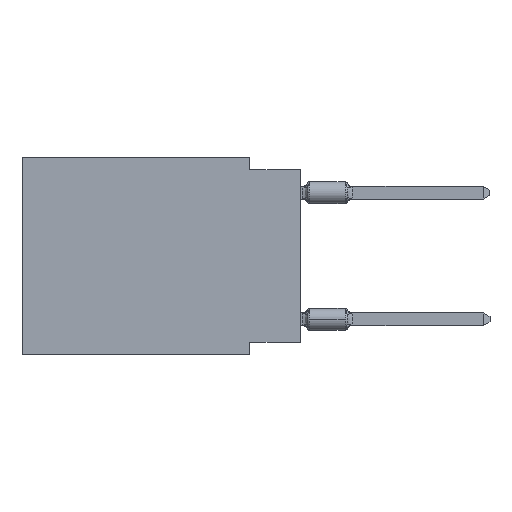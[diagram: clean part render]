
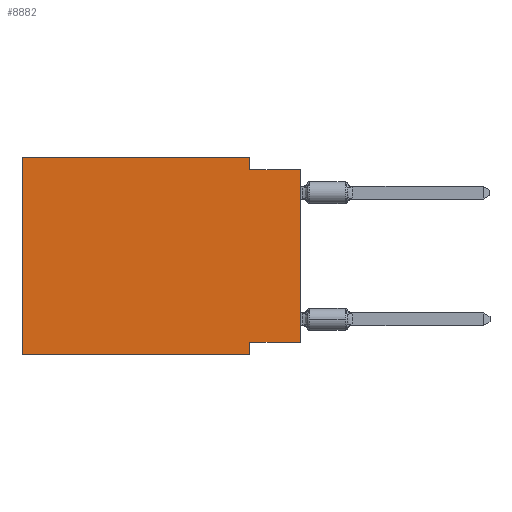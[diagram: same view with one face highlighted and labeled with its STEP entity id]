
A CAD part, left-side view. The second image highlights one B-rep face of the part: STEP entity #8882.
In plain terms, the highlighted planar face has unit normal (-1, 0, 0).
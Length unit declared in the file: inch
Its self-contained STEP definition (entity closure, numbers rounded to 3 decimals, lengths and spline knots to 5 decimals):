
#130 = EDGE_CURVE ( 'NONE', #8634, #6381, #14259, .T. ) ;
#194 = EDGE_CURVE ( 'NONE', #8634, #4099, #12026, .T. ) ;
#901 = EDGE_CURVE ( 'NONE', #6381, #3580, #13754, .T. ) ;
#1161 = VERTEX_POINT ( 'NONE', #1601 ) ;
#1203 = LINE ( 'NONE', #8480, #13628 ) ;
#1282 = EDGE_CURVE ( 'NONE', #3580, #2836, #10297, .T. ) ;
#1601 = CARTESIAN_POINT ( 'NONE',  ( 0., 0.1, -0.365 ) ) ;
#1873 = VECTOR ( 'NONE', #9549, 39.37008 ) ;
#1972 = ORIENTED_EDGE ( 'NONE', *, *, #6650, .F. ) ;
#2029 = VECTOR ( 'NONE', #4628, 39.37008 ) ;
#2389 = AXIS2_PLACEMENT_3D ( 'NONE', #9356, #9590, #9273 ) ;
#2646 = CARTESIAN_POINT ( 'NONE',  ( 0., 0., -0.025 ) ) ;
#2836 = VERTEX_POINT ( 'NONE', #4512 ) ;
#3253 = DIRECTION ( 'NONE',  ( 0., 0., 1. ) ) ;
#3470 = VECTOR ( 'NONE', #3253, 39.37008 ) ;
#3580 = VERTEX_POINT ( 'NONE', #4321 ) ;
#4099 = VERTEX_POINT ( 'NONE', #14002 ) ;
#4321 = CARTESIAN_POINT ( 'NONE',  ( 0., 0.1, 0. ) ) ;
#4357 = CARTESIAN_POINT ( 'NONE',  ( 0., 0.55, 0. ) ) ;
#4377 = CARTESIAN_POINT ( 'NONE',  ( 0., 0., 0. ) ) ;
#4426 = VERTEX_POINT ( 'NONE', #13079 ) ;
#4475 = CARTESIAN_POINT ( 'NONE',  ( 0., 0.1, 0. ) ) ;
#4512 = CARTESIAN_POINT ( 'NONE',  ( 0., 0.1, -0.025 ) ) ;
#4529 = VECTOR ( 'NONE', #9880, 39.37008 ) ;
#4559 = EDGE_CURVE ( 'NONE', #2836, #14212, #1203, .T. ) ;
#4628 = DIRECTION ( 'NONE',  ( 0., -1., 0. ) ) ;
#5025 = CARTESIAN_POINT ( 'NONE',  ( 0., 0.1, -0.39 ) ) ;
#5180 = EDGE_CURVE ( 'NONE', #4426, #14212, #15521, .T. ) ;
#5213 = EDGE_LOOP ( 'NONE', ( #6523, #6225, #11697, #9829, #9132, #13107, #1972, #9410 ) ) ;
#6225 = ORIENTED_EDGE ( 'NONE', *, *, #4559, .F. ) ;
#6381 = VERTEX_POINT ( 'NONE', #9246 ) ;
#6523 = ORIENTED_EDGE ( 'NONE', *, *, #5180, .T. ) ;
#6650 = EDGE_CURVE ( 'NONE', #1161, #4099, #11060, .T. ) ;
#7401 = VECTOR ( 'NONE', #12105, 39.37008 ) ;
#8480 = CARTESIAN_POINT ( 'NONE',  ( 0., 0., -0.025 ) ) ;
#8535 = CARTESIAN_POINT ( 'NONE',  ( 0., 0.55, 0. ) ) ;
#8634 = VERTEX_POINT ( 'NONE', #14031 ) ;
#8882 = ADVANCED_FACE ( 'NONE', ( #15630 ), #15552, .F. ) ;
#9132 = ORIENTED_EDGE ( 'NONE', *, *, #130, .F. ) ;
#9220 = DIRECTION ( 'NONE',  ( 0., -1., 0. ) ) ;
#9246 = CARTESIAN_POINT ( 'NONE',  ( 0., 0.55, 0. ) ) ;
#9273 = DIRECTION ( 'NONE',  ( 0., 0., -1. ) ) ;
#9356 = CARTESIAN_POINT ( 'NONE',  ( 0., 0.55, 0. ) ) ;
#9410 = ORIENTED_EDGE ( 'NONE', *, *, #10706, .F. ) ;
#9549 = DIRECTION ( 'NONE',  ( 0., 1., 0. ) ) ;
#9590 = DIRECTION ( 'NONE',  ( 1., 0., 0. ) ) ;
#9829 = ORIENTED_EDGE ( 'NONE', *, *, #901, .F. ) ;
#9880 = DIRECTION ( 'NONE',  ( 0., 0., -1. ) ) ;
#10297 = LINE ( 'NONE', #4475, #13783 ) ;
#10448 = VECTOR ( 'NONE', #9220, 39.37008 ) ;
#10706 = EDGE_CURVE ( 'NONE', #4426, #1161, #14405, .T. ) ;
#11060 = LINE ( 'NONE', #5025, #4529 ) ;
#11645 = DIRECTION ( 'NONE',  ( 0., 0., -1. ) ) ;
#11697 = ORIENTED_EDGE ( 'NONE', *, *, #1282, .F. ) ;
#12026 = LINE ( 'NONE', #14508, #2029 ) ;
#12105 = DIRECTION ( 'NONE',  ( 0., 0., 1. ) ) ;
#12790 = CARTESIAN_POINT ( 'NONE',  ( 0., 0., -0.365 ) ) ;
#13079 = CARTESIAN_POINT ( 'NONE',  ( 0., 0., -0.365 ) ) ;
#13107 = ORIENTED_EDGE ( 'NONE', *, *, #194, .T. ) ;
#13320 = DIRECTION ( 'NONE',  ( 0., -1., 0. ) ) ;
#13628 = VECTOR ( 'NONE', #13320, 39.37008 ) ;
#13754 = LINE ( 'NONE', #4357, #10448 ) ;
#13783 = VECTOR ( 'NONE', #11645, 39.37008 ) ;
#14002 = CARTESIAN_POINT ( 'NONE',  ( 0., 0.1, -0.39 ) ) ;
#14031 = CARTESIAN_POINT ( 'NONE',  ( 0., 0.55, -0.39 ) ) ;
#14212 = VERTEX_POINT ( 'NONE', #2646 ) ;
#14259 = LINE ( 'NONE', #8535, #7401 ) ;
#14405 = LINE ( 'NONE', #12790, #1873 ) ;
#14508 = CARTESIAN_POINT ( 'NONE',  ( 0., 0.55, -0.39 ) ) ;
#15521 = LINE ( 'NONE', #4377, #3470 ) ;
#15552 = PLANE ( 'NONE',  #2389 ) ;
#15630 = FACE_OUTER_BOUND ( 'NONE', #5213, .T. ) ;
